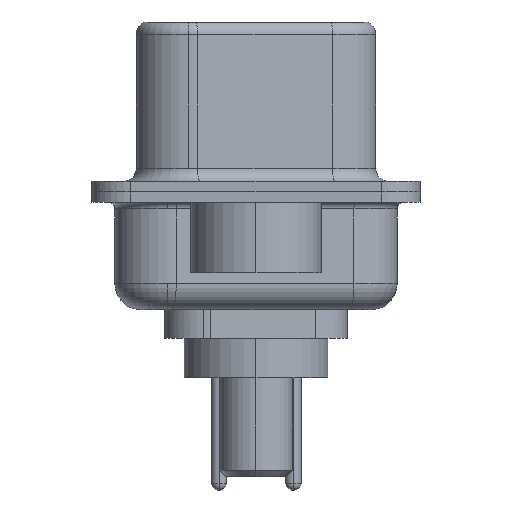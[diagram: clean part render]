
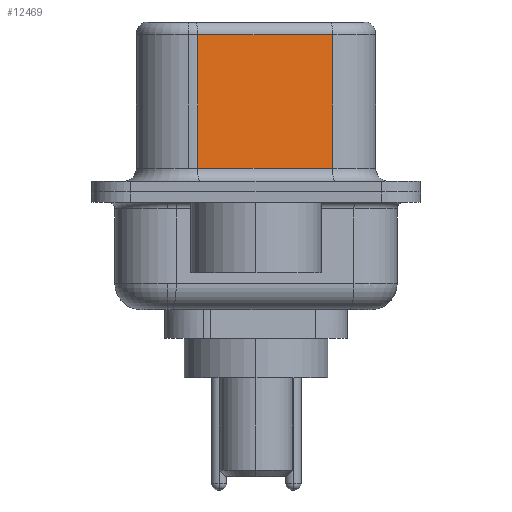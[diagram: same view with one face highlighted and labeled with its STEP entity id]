
A CAD part, left-side view. The second image highlights one B-rep face of the part: STEP entity #12469.
In plain terms, the highlighted planar face has unit normal (-0.985, -0.174, 0).
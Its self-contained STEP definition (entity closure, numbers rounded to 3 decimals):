
#130 = DIRECTION ( 'NONE',  ( 0., 0., -1. ) ) ;
#147 = CARTESIAN_POINT ( 'NONE',  ( 4.565, -2.927, 6.52 ) ) ;
#1521 = EDGE_CURVE ( 'NONE', #2765, #4409, #13713, .T. ) ;
#1575 = EDGE_CURVE ( 'NONE', #10163, #4409, #12606, .T. ) ;
#1817 = VERTEX_POINT ( 'NONE', #12048 ) ;
#2752 = DIRECTION ( 'NONE',  ( -0.174, 0.985, 0. ) ) ;
#2765 = VERTEX_POINT ( 'NONE', #2869 ) ;
#2795 = ORIENTED_EDGE ( 'NONE', *, *, #1575, .T. ) ;
#2864 = CARTESIAN_POINT ( 'NONE',  ( 3.655, 2.233, 0.9 ) ) ;
#2869 = CARTESIAN_POINT ( 'NONE',  ( 4.565, -2.927, 6.02 ) ) ;
#3303 = VECTOR ( 'NONE', #3679, 1000. ) ;
#3457 = CARTESIAN_POINT ( 'NONE',  ( 4.565, -2.927, 6.02 ) ) ;
#3679 = DIRECTION ( 'NONE',  ( 0.174, -0.985, 0. ) ) ;
#3720 = CARTESIAN_POINT ( 'NONE',  ( 3.655, 2.233, 6.52 ) ) ;
#3878 = DIRECTION ( 'NONE',  ( 0., 0., -1. ) ) ;
#4153 = LINE ( 'NONE', #3720, #7042 ) ;
#4194 = CARTESIAN_POINT ( 'NONE',  ( 4.565, -2.927, 0.9 ) ) ;
#4260 = EDGE_LOOP ( 'NONE', ( #6809, #9820, #13406, #2795 ) ) ;
#4409 = VERTEX_POINT ( 'NONE', #4194 ) ;
#4495 = LINE ( 'NONE', #3457, #10194 ) ;
#5040 = CARTESIAN_POINT ( 'NONE',  ( 4.565, -2.927, 6.52 ) ) ;
#5421 = FACE_OUTER_BOUND ( 'NONE', #4260, .T. ) ;
#6809 = ORIENTED_EDGE ( 'NONE', *, *, #1521, .F. ) ;
#7042 = VECTOR ( 'NONE', #130, 1000. ) ;
#7357 = VECTOR ( 'NONE', #3878, 1000. ) ;
#7390 = PLANE ( 'NONE',  #7517 ) ;
#7517 = AXIS2_PLACEMENT_3D ( 'NONE', #147, #10013, #2752 ) ;
#9820 = ORIENTED_EDGE ( 'NONE', *, *, #12250, .T. ) ;
#10013 = DIRECTION ( 'NONE',  ( 0.985, 0.174, 0. ) ) ;
#10163 = VERTEX_POINT ( 'NONE', #2864 ) ;
#10194 = VECTOR ( 'NONE', #10720, 1000. ) ;
#10720 = DIRECTION ( 'NONE',  ( -0.174, 0.985, 0. ) ) ;
#11143 = EDGE_CURVE ( 'NONE', #1817, #10163, #4153, .T. ) ;
#12048 = CARTESIAN_POINT ( 'NONE',  ( 3.655, 2.233, 6.02 ) ) ;
#12250 = EDGE_CURVE ( 'NONE', #2765, #1817, #4495, .T. ) ;
#12469 = ADVANCED_FACE ( 'NONE', ( #5421 ), #7390, .F. ) ;
#12606 = LINE ( 'NONE', #13183, #3303 ) ;
#13183 = CARTESIAN_POINT ( 'NONE',  ( 4.565, -2.927, 0.9 ) ) ;
#13406 = ORIENTED_EDGE ( 'NONE', *, *, #11143, .T. ) ;
#13713 = LINE ( 'NONE', #5040, #7357 ) ;
